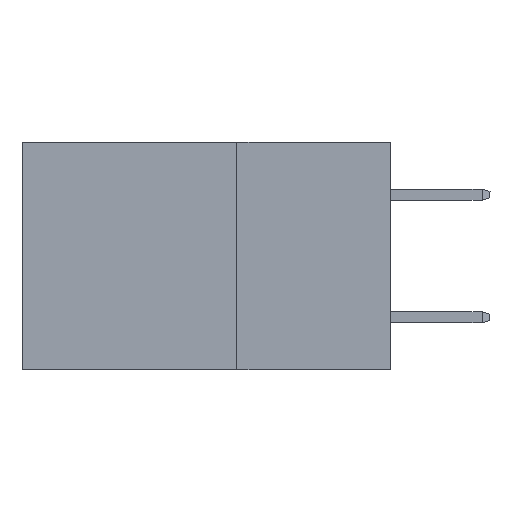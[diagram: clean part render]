
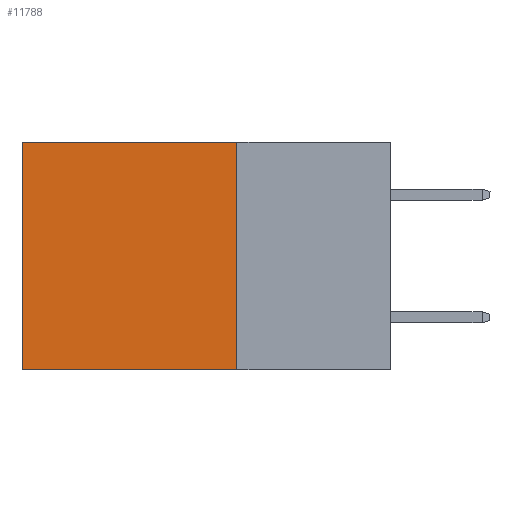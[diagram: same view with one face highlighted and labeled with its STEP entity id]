
A CAD part, left-side view. The second image highlights one B-rep face of the part: STEP entity #11788.
In plain terms, the highlighted planar face has unit normal (-1, 0, 0).
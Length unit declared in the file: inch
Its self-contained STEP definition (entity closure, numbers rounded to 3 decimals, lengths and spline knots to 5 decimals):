
#62 = CARTESIAN_POINT ( 'NONE',  ( 0.2875, 0.6, 0. ) ) ;
#333 = LINE ( 'NONE', #1259, #5840 ) ;
#1104 = DIRECTION ( 'NONE',  ( 0., 0., -1. ) ) ;
#1156 = CARTESIAN_POINT ( 'NONE',  ( 0.2875, 0.25, 0. ) ) ;
#1259 = CARTESIAN_POINT ( 'NONE',  ( 0.2875, 0.25, -0.37 ) ) ;
#1730 = ORIENTED_EDGE ( 'NONE', *, *, #4027, .T. ) ;
#1783 = CARTESIAN_POINT ( 'NONE',  ( 0.2875, 0.25, 0. ) ) ;
#1826 = DIRECTION ( 'NONE',  ( 1., 0., 0. ) ) ;
#2018 = VECTOR ( 'NONE', #7478, 39.37008 ) ;
#2386 = DIRECTION ( 'NONE',  ( 0., 1., 0. ) ) ;
#2436 = EDGE_CURVE ( 'NONE', #8369, #8703, #3987, .T. ) ;
#2888 = CARTESIAN_POINT ( 'NONE',  ( 0.2875, 0.25, 0. ) ) ;
#2958 = EDGE_CURVE ( 'NONE', #8703, #7410, #333, .T. ) ;
#2972 = EDGE_LOOP ( 'NONE', ( #11221, #11438, #4186, #1730 ) ) ;
#3232 = FACE_OUTER_BOUND ( 'NONE', #2972, .T. ) ;
#3987 = LINE ( 'NONE', #1156, #9751 ) ;
#4027 = EDGE_CURVE ( 'NONE', #8369, #9803, #12045, .T. ) ;
#4186 = ORIENTED_EDGE ( 'NONE', *, *, #2436, .F. ) ;
#5060 = PLANE ( 'NONE',  #13941 ) ;
#5840 = VECTOR ( 'NONE', #2386, 39.37008 ) ;
#6305 = VECTOR ( 'NONE', #12896, 39.37008 ) ;
#7410 = VERTEX_POINT ( 'NONE', #11960 ) ;
#7478 = DIRECTION ( 'NONE',  ( 0., 0., -1. ) ) ;
#7768 = LINE ( 'NONE', #13904, #2018 ) ;
#7871 = CARTESIAN_POINT ( 'NONE',  ( 0.2875, 0.25, -0.37 ) ) ;
#8369 = VERTEX_POINT ( 'NONE', #2888 ) ;
#8623 = CARTESIAN_POINT ( 'NONE',  ( 0.2875, 0.25, 0. ) ) ;
#8703 = VERTEX_POINT ( 'NONE', #7871 ) ;
#9401 = DIRECTION ( 'NONE',  ( 0., 0., -1. ) ) ;
#9751 = VECTOR ( 'NONE', #1104, 39.37008 ) ;
#9803 = VERTEX_POINT ( 'NONE', #62 ) ;
#11221 = ORIENTED_EDGE ( 'NONE', *, *, #12514, .T. ) ;
#11438 = ORIENTED_EDGE ( 'NONE', *, *, #2958, .F. ) ;
#11788 = ADVANCED_FACE ( 'NONE', ( #3232 ), #5060, .F. ) ;
#11960 = CARTESIAN_POINT ( 'NONE',  ( 0.2875, 0.6, -0.37 ) ) ;
#12045 = LINE ( 'NONE', #8623, #6305 ) ;
#12514 = EDGE_CURVE ( 'NONE', #9803, #7410, #7768, .T. ) ;
#12896 = DIRECTION ( 'NONE',  ( 0., 1., 0. ) ) ;
#13904 = CARTESIAN_POINT ( 'NONE',  ( 0.2875, 0.6, 0. ) ) ;
#13941 = AXIS2_PLACEMENT_3D ( 'NONE', #1783, #1826, #9401 ) ;
